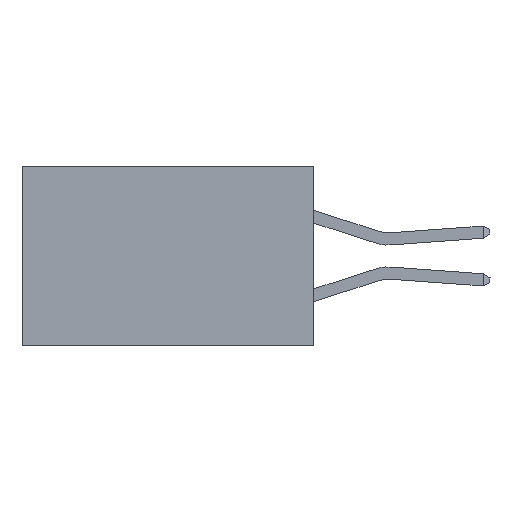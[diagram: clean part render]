
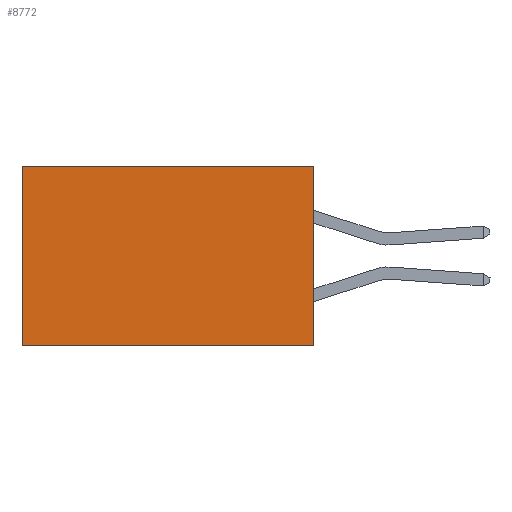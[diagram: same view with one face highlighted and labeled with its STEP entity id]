
A CAD part, left-side view. The second image highlights one B-rep face of the part: STEP entity #8772.
In plain terms, the highlighted planar face has unit normal (-1, 0, 0).
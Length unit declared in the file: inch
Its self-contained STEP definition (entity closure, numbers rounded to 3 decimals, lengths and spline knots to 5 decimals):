
#268 = EDGE_CURVE ( 'NONE', #14924, #19786, #7311, .T. ) ;
#375 = DIRECTION ( 'NONE',  ( 0., 0., -1. ) ) ;
#479 = VERTEX_POINT ( 'NONE', #740 ) ;
#740 = CARTESIAN_POINT ( 'NONE',  ( 0.2875, 0., -0.37 ) ) ;
#804 = PLANE ( 'NONE',  #5046 ) ;
#846 = CARTESIAN_POINT ( 'NONE',  ( 0.2875, 0., 0. ) ) ;
#1039 = VECTOR ( 'NONE', #5881, 39.37008 ) ;
#2457 = DIRECTION ( 'NONE',  ( 1., 0., 0. ) ) ;
#5046 = AXIS2_PLACEMENT_3D ( 'NONE', #10385, #2457, #13541 ) ;
#5048 = EDGE_CURVE ( 'NONE', #19786, #12008, #12170, .T. ) ;
#5274 = DIRECTION ( 'NONE',  ( 0., 1., 0. ) ) ;
#5728 = ORIENTED_EDGE ( 'NONE', *, *, #17379, .F. ) ;
#5822 = ORIENTED_EDGE ( 'NONE', *, *, #5048, .T. ) ;
#5881 = DIRECTION ( 'NONE',  ( 0., 1., 0. ) ) ;
#6031 = EDGE_CURVE ( 'NONE', #14924, #479, #13113, .T. ) ;
#7311 = LINE ( 'NONE', #12917, #18746 ) ;
#8772 = ADVANCED_FACE ( 'NONE', ( #11051 ), #804, .F. ) ;
#9350 = CARTESIAN_POINT ( 'NONE',  ( 0.2875, 0.6, 0. ) ) ;
#9994 = CARTESIAN_POINT ( 'NONE',  ( 0.2875, 0., 0. ) ) ;
#10385 = CARTESIAN_POINT ( 'NONE',  ( 0.2875, 0., 0. ) ) ;
#10470 = CARTESIAN_POINT ( 'NONE',  ( 0.2875, 0., -0.37 ) ) ;
#11051 = FACE_OUTER_BOUND ( 'NONE', #17709, .T. ) ;
#11180 = VECTOR ( 'NONE', #12485, 39.37008 ) ;
#11278 = ORIENTED_EDGE ( 'NONE', *, *, #6031, .F. ) ;
#12008 = VERTEX_POINT ( 'NONE', #15746 ) ;
#12170 = LINE ( 'NONE', #9350, #11180 ) ;
#12485 = DIRECTION ( 'NONE',  ( 0., 0., -1. ) ) ;
#12917 = CARTESIAN_POINT ( 'NONE',  ( 0.2875, 0., 0. ) ) ;
#13113 = LINE ( 'NONE', #9994, #13607 ) ;
#13541 = DIRECTION ( 'NONE',  ( 0., 0., -1. ) ) ;
#13607 = VECTOR ( 'NONE', #375, 39.37008 ) ;
#14008 = ORIENTED_EDGE ( 'NONE', *, *, #268, .T. ) ;
#14924 = VERTEX_POINT ( 'NONE', #846 ) ;
#15746 = CARTESIAN_POINT ( 'NONE',  ( 0.2875, 0.6, -0.37 ) ) ;
#17379 = EDGE_CURVE ( 'NONE', #479, #12008, #17866, .T. ) ;
#17401 = CARTESIAN_POINT ( 'NONE',  ( 0.2875, 0.6, 0. ) ) ;
#17709 = EDGE_LOOP ( 'NONE', ( #5822, #5728, #11278, #14008 ) ) ;
#17866 = LINE ( 'NONE', #10470, #1039 ) ;
#18746 = VECTOR ( 'NONE', #5274, 39.37008 ) ;
#19786 = VERTEX_POINT ( 'NONE', #17401 ) ;
